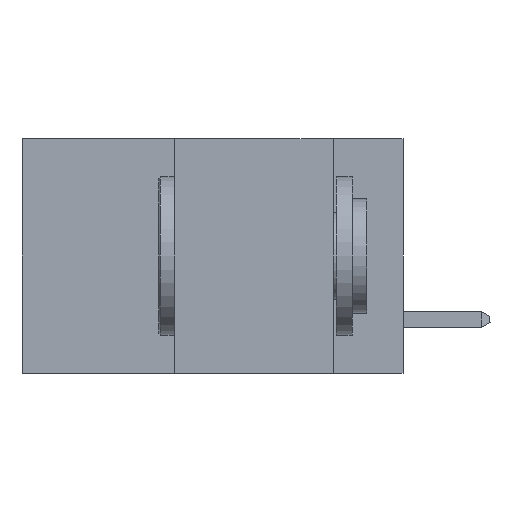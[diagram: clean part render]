
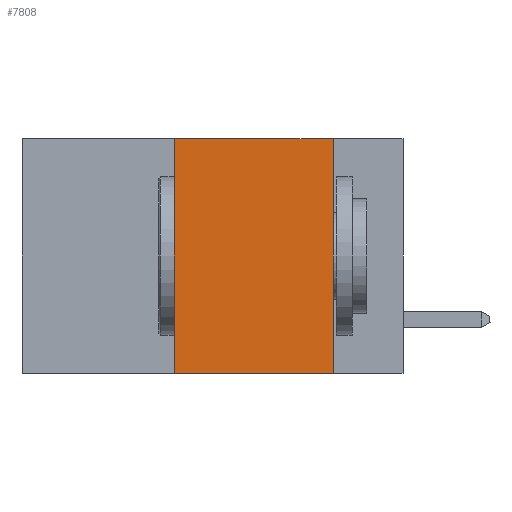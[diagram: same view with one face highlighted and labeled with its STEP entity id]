
A CAD part, left-side view. The second image highlights one B-rep face of the part: STEP entity #7808.
In plain terms, the highlighted planar face has unit normal (-1, 0, 0).
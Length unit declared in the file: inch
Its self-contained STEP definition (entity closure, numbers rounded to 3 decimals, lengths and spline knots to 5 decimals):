
#186 = EDGE_LOOP ( 'NONE', ( #32775, #10609, #35050, #21214 ) ) ;
#970 = EDGE_CURVE ( 'NONE', #41604, #16803, #1397, .T. ) ;
#1149 = DIRECTION ( 'NONE',  ( 1., 0., 0. ) ) ;
#1397 = LINE ( 'NONE', #36123, #27612 ) ;
#3282 = CARTESIAN_POINT ( 'NONE',  ( 0., 0.6, -0.37 ) ) ;
#4336 = LINE ( 'NONE', #38535, #20439 ) ;
#4942 = DIRECTION ( 'NONE',  ( 0., -1., 0. ) ) ;
#5429 = LINE ( 'NONE', #7776, #38641 ) ;
#6647 = EDGE_CURVE ( 'NONE', #36575, #40719, #4336, .T. ) ;
#6778 = CARTESIAN_POINT ( 'NONE',  ( 0., 0.36, -0.37 ) ) ;
#7776 = CARTESIAN_POINT ( 'NONE',  ( 0., 0.6, 0. ) ) ;
#7808 = ADVANCED_FACE ( 'NONE', ( #22121 ), #23827, .F. ) ;
#8564 = AXIS2_PLACEMENT_3D ( 'NONE', #16932, #1149, #10708 ) ;
#10609 = ORIENTED_EDGE ( 'NONE', *, *, #26723, .F. ) ;
#10708 = DIRECTION ( 'NONE',  ( 0., 0., -1. ) ) ;
#10853 = CARTESIAN_POINT ( 'NONE',  ( 0., 0.11, -0.37 ) ) ;
#15896 = DIRECTION ( 'NONE',  ( 0., 0., 1. ) ) ;
#16146 = CARTESIAN_POINT ( 'NONE',  ( 0., 0.36, 0. ) ) ;
#16410 = DIRECTION ( 'NONE',  ( 0., 0., -1. ) ) ;
#16803 = VERTEX_POINT ( 'NONE', #10853 ) ;
#16932 = CARTESIAN_POINT ( 'NONE',  ( 0., 0.6, 0. ) ) ;
#17740 = EDGE_CURVE ( 'NONE', #36575, #16803, #22315, .T. ) ;
#18467 = CARTESIAN_POINT ( 'NONE',  ( 0., 0.11, 0. ) ) ;
#20439 = VECTOR ( 'NONE', #15896, 39.37008 ) ;
#21214 = ORIENTED_EDGE ( 'NONE', *, *, #17740, .T. ) ;
#22121 = FACE_OUTER_BOUND ( 'NONE', #186, .T. ) ;
#22315 = LINE ( 'NONE', #3282, #33397 ) ;
#22698 = DIRECTION ( 'NONE',  ( 0., -1., 0. ) ) ;
#23827 = PLANE ( 'NONE',  #8564 ) ;
#26723 = EDGE_CURVE ( 'NONE', #40719, #41604, #5429, .T. ) ;
#27612 = VECTOR ( 'NONE', #16410, 39.37008 ) ;
#32775 = ORIENTED_EDGE ( 'NONE', *, *, #970, .F. ) ;
#33397 = VECTOR ( 'NONE', #22698, 39.37008 ) ;
#35050 = ORIENTED_EDGE ( 'NONE', *, *, #6647, .F. ) ;
#36123 = CARTESIAN_POINT ( 'NONE',  ( 0., 0.11, 0. ) ) ;
#36575 = VERTEX_POINT ( 'NONE', #6778 ) ;
#38535 = CARTESIAN_POINT ( 'NONE',  ( 0., 0.36, 0. ) ) ;
#38641 = VECTOR ( 'NONE', #4942, 39.37008 ) ;
#40719 = VERTEX_POINT ( 'NONE', #16146 ) ;
#41604 = VERTEX_POINT ( 'NONE', #18467 ) ;
